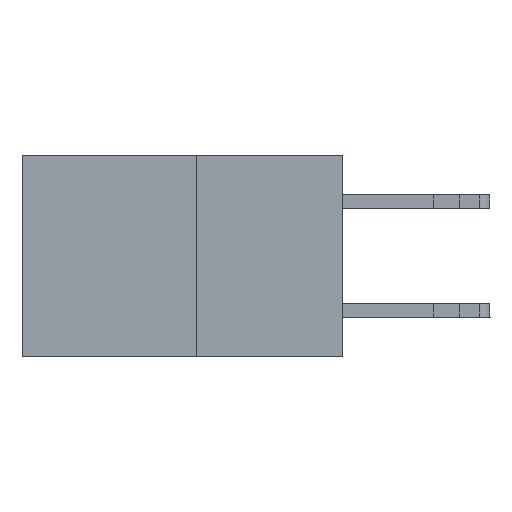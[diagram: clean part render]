
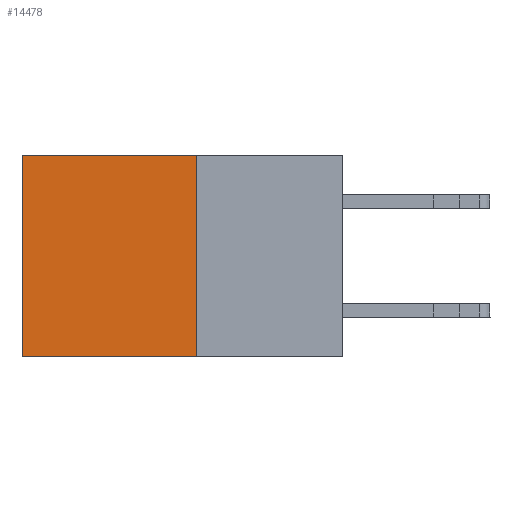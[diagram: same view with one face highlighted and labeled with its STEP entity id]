
A CAD part, left-side view. The second image highlights one B-rep face of the part: STEP entity #14478.
In plain terms, the highlighted planar face has unit normal (-1, 0, 0).
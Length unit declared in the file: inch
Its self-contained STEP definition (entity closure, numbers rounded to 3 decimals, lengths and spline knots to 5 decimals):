
#394 = ORIENTED_EDGE ( 'NONE', *, *, #22251, .F. ) ;
#546 = VECTOR ( 'NONE', #20490, 39.37008 ) ;
#1315 = CARTESIAN_POINT ( 'NONE',  ( 0.277, 0.27, -0.37 ) ) ;
#1714 = DIRECTION ( 'NONE',  ( 0., 0., -1. ) ) ;
#2072 = EDGE_CURVE ( 'NONE', #12420, #17576, #14551, .T. ) ;
#3196 = DIRECTION ( 'NONE',  ( 0., 1., 0. ) ) ;
#4839 = CARTESIAN_POINT ( 'NONE',  ( 0.277, 0.59, -0.37 ) ) ;
#4841 = CARTESIAN_POINT ( 'NONE',  ( 0.277, 0.27, 0. ) ) ;
#5081 = VERTEX_POINT ( 'NONE', #12945 ) ;
#5377 = LINE ( 'NONE', #1315, #14021 ) ;
#6902 = LINE ( 'NONE', #17407, #15469 ) ;
#8246 = VECTOR ( 'NONE', #15159, 39.37008 ) ;
#9454 = ORIENTED_EDGE ( 'NONE', *, *, #15616, .F. ) ;
#9530 = AXIS2_PLACEMENT_3D ( 'NONE', #10489, #12178, #1714 ) ;
#10489 = CARTESIAN_POINT ( 'NONE',  ( 0.277, 0.27, -0.37 ) ) ;
#10808 = ORIENTED_EDGE ( 'NONE', *, *, #10902, .T. ) ;
#10902 = EDGE_CURVE ( 'NONE', #5081, #12420, #21697, .T. ) ;
#12178 = DIRECTION ( 'NONE',  ( 1., 0., 0. ) ) ;
#12420 = VERTEX_POINT ( 'NONE', #20581 ) ;
#12945 = CARTESIAN_POINT ( 'NONE',  ( 0.277, 0.27, 0. ) ) ;
#13193 = FACE_OUTER_BOUND ( 'NONE', #19394, .T. ) ;
#13555 = VERTEX_POINT ( 'NONE', #16945 ) ;
#14021 = VECTOR ( 'NONE', #3196, 39.37008 ) ;
#14478 = ADVANCED_FACE ( 'NONE', ( #13193 ), #20552, .F. ) ;
#14551 = LINE ( 'NONE', #19975, #546 ) ;
#15159 = DIRECTION ( 'NONE',  ( 0., 1., 0. ) ) ;
#15469 = VECTOR ( 'NONE', #19114, 39.37008 ) ;
#15616 = EDGE_CURVE ( 'NONE', #13555, #17576, #5377, .T. ) ;
#16945 = CARTESIAN_POINT ( 'NONE',  ( 0.277, 0.27, -0.37 ) ) ;
#17407 = CARTESIAN_POINT ( 'NONE',  ( 0.277, 0.27, -0.37 ) ) ;
#17576 = VERTEX_POINT ( 'NONE', #4839 ) ;
#18940 = ORIENTED_EDGE ( 'NONE', *, *, #2072, .T. ) ;
#19114 = DIRECTION ( 'NONE',  ( 0., 0., -1. ) ) ;
#19394 = EDGE_LOOP ( 'NONE', ( #18940, #9454, #394, #10808 ) ) ;
#19975 = CARTESIAN_POINT ( 'NONE',  ( 0.277, 0.59, -0.37 ) ) ;
#20490 = DIRECTION ( 'NONE',  ( 0., 0., -1. ) ) ;
#20552 = PLANE ( 'NONE',  #9530 ) ;
#20581 = CARTESIAN_POINT ( 'NONE',  ( 0.277, 0.59, 0. ) ) ;
#21697 = LINE ( 'NONE', #4841, #8246 ) ;
#22251 = EDGE_CURVE ( 'NONE', #5081, #13555, #6902, .T. ) ;
